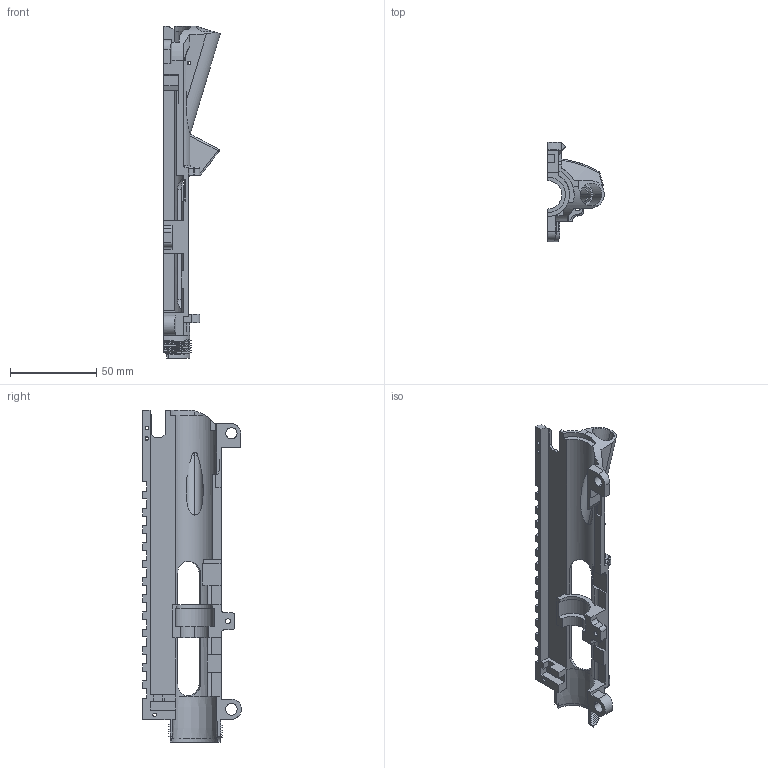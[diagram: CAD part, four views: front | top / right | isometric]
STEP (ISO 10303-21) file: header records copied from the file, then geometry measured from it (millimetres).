
FILE_DESCRIPTION (( 'STEP AP203' ), '1' );
FILE_NAME ('vr15_upper_r.STEP', '2021-12-29T04:24:33', ( '' ), ( '' ), 'SwSTEP 2.0', 'SolidWorks 2015', '' );
FILE_SCHEMA (( 'CONFIG_CONTROL_DESIGN' ));
Length unit declared in the file: millimetre
Products named in the file (1): vr15_upper_r
Bounding box: 32.84 x 57.3 x 192.5 mm (x, y, z)
Volume: 37596.3 mm3; surface area: 28642.5 mm2
Topology: 1 solids, 1 shells, 335 faces, 941 edges, 606 vertices
Faces by surface type: plane 195, cylinder 104, bspline 24, torus 7, sphere 4, cone 1
Entity records: 14058 total; most frequent: CARTESIAN_POINT 5592, ORIENTED_EDGE 1876, DIRECTION 1614, EDGE_CURVE 938, VERTEX_POINT 604, LINE 590, VECTOR 590, AXIS2_PLACEMENT_3D 512
